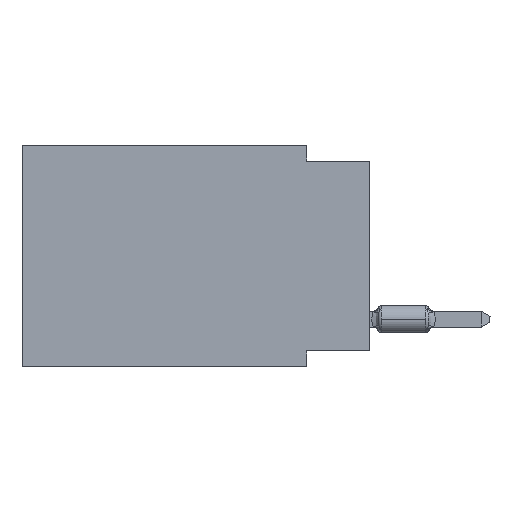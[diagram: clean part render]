
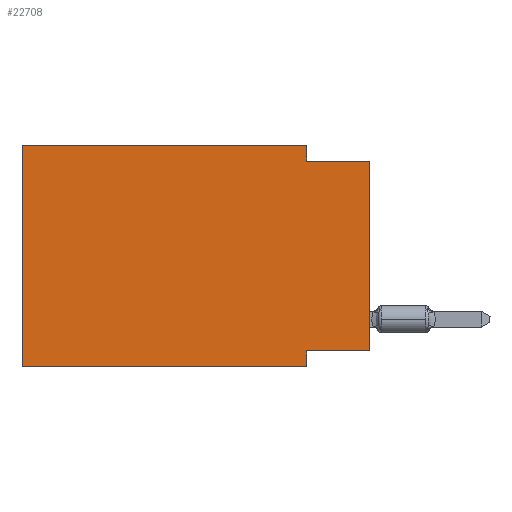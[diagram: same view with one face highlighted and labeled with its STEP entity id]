
A CAD part, left-side view. The second image highlights one B-rep face of the part: STEP entity #22708.
In plain terms, the highlighted planar face has unit normal (-1, 0, 0).
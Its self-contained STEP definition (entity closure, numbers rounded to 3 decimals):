
#509 = DIRECTION ( 'NONE',  ( 0., -1., 0. ) ) ;
#865 = EDGE_CURVE ( 'NONE', #12982, #1234, #23842, .T. ) ;
#1234 = VERTEX_POINT ( 'NONE', #4410 ) ;
#1468 = CARTESIAN_POINT ( 'NONE',  ( 0., 2.54, -8.89 ) ) ;
#1602 = CARTESIAN_POINT ( 'NONE',  ( 0., 2.54, -0.635 ) ) ;
#1872 = VECTOR ( 'NONE', #22749, 1000. ) ;
#1919 = CARTESIAN_POINT ( 'NONE',  ( 0., 13.97, -8.89 ) ) ;
#2232 = CARTESIAN_POINT ( 'NONE',  ( 0., 13.97, -8.89 ) ) ;
#3010 = LINE ( 'NONE', #14821, #5072 ) ;
#4152 = EDGE_CURVE ( 'NONE', #23303, #17989, #7079, .T. ) ;
#4410 = CARTESIAN_POINT ( 'NONE',  ( 0., 13.97, 0. ) ) ;
#4665 = EDGE_CURVE ( 'NONE', #1234, #23303, #6422, .T. ) ;
#4692 = VECTOR ( 'NONE', #14458, 1000. ) ;
#5063 = DIRECTION ( 'NONE',  ( 0., 0., -1. ) ) ;
#5072 = VECTOR ( 'NONE', #5063, 1000. ) ;
#5216 = CARTESIAN_POINT ( 'NONE',  ( 0., 0., -0.635 ) ) ;
#6032 = ORIENTED_EDGE ( 'NONE', *, *, #865, .F. ) ;
#6161 = CARTESIAN_POINT ( 'NONE',  ( 0., 0., 0. ) ) ;
#6422 = LINE ( 'NONE', #8463, #8858 ) ;
#7079 = LINE ( 'NONE', #24420, #1872 ) ;
#8302 = ORIENTED_EDGE ( 'NONE', *, *, #24131, .F. ) ;
#8463 = CARTESIAN_POINT ( 'NONE',  ( 0., 13.97, 0. ) ) ;
#8489 = LINE ( 'NONE', #14655, #11148 ) ;
#8509 = DIRECTION ( 'NONE',  ( 0., 0., -1. ) ) ;
#8666 = VECTOR ( 'NONE', #13999, 1000. ) ;
#8858 = VECTOR ( 'NONE', #15923, 1000. ) ;
#10151 = VECTOR ( 'NONE', #20035, 1000. ) ;
#11148 = VECTOR ( 'NONE', #22362, 1000. ) ;
#11575 = CARTESIAN_POINT ( 'NONE',  ( 0., 0., -8.255 ) ) ;
#11744 = AXIS2_PLACEMENT_3D ( 'NONE', #16487, #14549, #8509 ) ;
#12073 = EDGE_CURVE ( 'NONE', #12982, #17816, #17848, .T. ) ;
#12285 = ORIENTED_EDGE ( 'NONE', *, *, #21149, .F. ) ;
#12858 = VERTEX_POINT ( 'NONE', #5216 ) ;
#12982 = VERTEX_POINT ( 'NONE', #2232 ) ;
#13999 = DIRECTION ( 'NONE',  ( 0., 0., 1. ) ) ;
#14380 = CARTESIAN_POINT ( 'NONE',  ( 0., 0., -0.635 ) ) ;
#14458 = DIRECTION ( 'NONE',  ( 0., 0., 1. ) ) ;
#14549 = DIRECTION ( 'NONE',  ( 1., 0., 0. ) ) ;
#14655 = CARTESIAN_POINT ( 'NONE',  ( 0., 0., -8.255 ) ) ;
#14821 = CARTESIAN_POINT ( 'NONE',  ( 0., 2.54, -8.89 ) ) ;
#14849 = VECTOR ( 'NONE', #509, 1000. ) ;
#15923 = DIRECTION ( 'NONE',  ( 0., -1., 0. ) ) ;
#16229 = FACE_OUTER_BOUND ( 'NONE', #18907, .T. ) ;
#16413 = ORIENTED_EDGE ( 'NONE', *, *, #16798, .F. ) ;
#16487 = CARTESIAN_POINT ( 'NONE',  ( 0., 13.97, 0. ) ) ;
#16798 = EDGE_CURVE ( 'NONE', #18316, #20642, #8489, .T. ) ;
#17816 = VERTEX_POINT ( 'NONE', #1468 ) ;
#17848 = LINE ( 'NONE', #1919, #10151 ) ;
#17989 = VERTEX_POINT ( 'NONE', #1602 ) ;
#18316 = VERTEX_POINT ( 'NONE', #11575 ) ;
#18907 = EDGE_LOOP ( 'NONE', ( #19052, #8302, #25126, #19122, #6032, #24103, #12285, #16413 ) ) ;
#19052 = ORIENTED_EDGE ( 'NONE', *, *, #23939, .T. ) ;
#19122 = ORIENTED_EDGE ( 'NONE', *, *, #4665, .F. ) ;
#20009 = CARTESIAN_POINT ( 'NONE',  ( 0., 2.54, -8.255 ) ) ;
#20035 = DIRECTION ( 'NONE',  ( 0., -1., 0. ) ) ;
#20642 = VERTEX_POINT ( 'NONE', #20009 ) ;
#21149 = EDGE_CURVE ( 'NONE', #20642, #17816, #3010, .T. ) ;
#21581 = LINE ( 'NONE', #6161, #8666 ) ;
#21820 = CARTESIAN_POINT ( 'NONE',  ( 0., 2.54, 0. ) ) ;
#22340 = LINE ( 'NONE', #14380, #14849 ) ;
#22362 = DIRECTION ( 'NONE',  ( 0., 1., 0. ) ) ;
#22708 = ADVANCED_FACE ( 'NONE', ( #16229 ), #24058, .F. ) ;
#22749 = DIRECTION ( 'NONE',  ( 0., 0., -1. ) ) ;
#23303 = VERTEX_POINT ( 'NONE', #21820 ) ;
#23842 = LINE ( 'NONE', #23968, #4692 ) ;
#23939 = EDGE_CURVE ( 'NONE', #18316, #12858, #21581, .T. ) ;
#23968 = CARTESIAN_POINT ( 'NONE',  ( 0., 13.97, 0. ) ) ;
#24058 = PLANE ( 'NONE',  #11744 ) ;
#24103 = ORIENTED_EDGE ( 'NONE', *, *, #12073, .T. ) ;
#24131 = EDGE_CURVE ( 'NONE', #17989, #12858, #22340, .T. ) ;
#24420 = CARTESIAN_POINT ( 'NONE',  ( 0., 2.54, 0. ) ) ;
#25126 = ORIENTED_EDGE ( 'NONE', *, *, #4152, .F. ) ;
